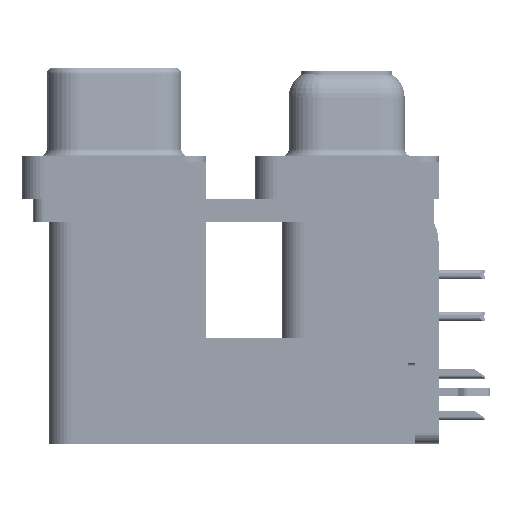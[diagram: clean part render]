
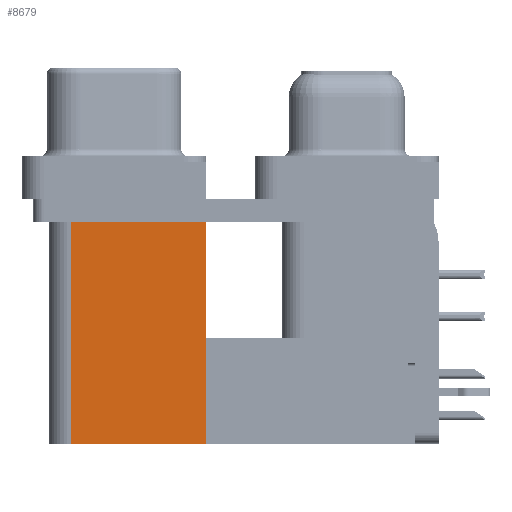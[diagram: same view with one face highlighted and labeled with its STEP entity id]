
A CAD part, left-side view. The second image highlights one B-rep face of the part: STEP entity #8679.
In plain terms, the highlighted planar face has unit normal (-1, 0, 0).
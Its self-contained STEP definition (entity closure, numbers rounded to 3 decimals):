
#277 = CARTESIAN_POINT ( 'NONE',  ( 3.79, 9.6, -2.5 ) ) ;
#1597 = AXIS2_PLACEMENT_3D ( 'NONE', #58110, #9900, #31339 ) ;
#2740 = ORIENTED_EDGE ( 'NONE', *, *, #32644, .F. ) ;
#8679 = ADVANCED_FACE ( 'NONE', ( #29939 ), #62696, .F. ) ;
#9900 = DIRECTION ( 'NONE',  ( 1., 0., 0. ) ) ;
#10101 = DIRECTION ( 'NONE',  ( 0., 1., 0. ) ) ;
#11709 = EDGE_CURVE ( 'NONE', #26536, #34856, #37534, .T. ) ;
#14113 = CARTESIAN_POINT ( 'NONE',  ( 3.79, 9.6, -2.5 ) ) ;
#20855 = VECTOR ( 'NONE', #66719, 1000. ) ;
#23496 = CARTESIAN_POINT ( 'NONE',  ( 3.79, 9.6, -19.2 ) ) ;
#23754 = LINE ( 'NONE', #45226, #20855 ) ;
#26536 = VERTEX_POINT ( 'NONE', #14113 ) ;
#27527 = EDGE_CURVE ( 'NONE', #42668, #34856, #57118, .T. ) ;
#29939 = FACE_OUTER_BOUND ( 'NONE', #42204, .T. ) ;
#31339 = DIRECTION ( 'NONE',  ( 0., 0., -1. ) ) ;
#31497 = EDGE_CURVE ( 'NONE', #40873, #26536, #32161, .T. ) ;
#32161 = LINE ( 'NONE', #53629, #51029 ) ;
#32644 = EDGE_CURVE ( 'NONE', #40873, #42668, #23754, .T. ) ;
#33054 = CARTESIAN_POINT ( 'NONE',  ( 3.79, 18.8, -2.5 ) ) ;
#34856 = VERTEX_POINT ( 'NONE', #33054 ) ;
#37534 = LINE ( 'NONE', #277, #57627 ) ;
#40873 = VERTEX_POINT ( 'NONE', #23496 ) ;
#42001 = ORIENTED_EDGE ( 'NONE', *, *, #11709, .T. ) ;
#42204 = EDGE_LOOP ( 'NONE', ( #42001, #47281, #2740, #51190 ) ) ;
#42366 = DIRECTION ( 'NONE',  ( 0., 0., 1. ) ) ;
#42668 = VERTEX_POINT ( 'NONE', #50528 ) ;
#45226 = CARTESIAN_POINT ( 'NONE',  ( 3.79, 9.6, -19.2 ) ) ;
#47281 = ORIENTED_EDGE ( 'NONE', *, *, #27527, .F. ) ;
#50528 = CARTESIAN_POINT ( 'NONE',  ( 3.79, 18.8, -19.2 ) ) ;
#51029 = VECTOR ( 'NONE', #42366, 1000. ) ;
#51190 = ORIENTED_EDGE ( 'NONE', *, *, #31497, .T. ) ;
#53629 = CARTESIAN_POINT ( 'NONE',  ( 3.79, 9.6, -19.2 ) ) ;
#56775 = CARTESIAN_POINT ( 'NONE',  ( 3.79, 18.8, -19.2 ) ) ;
#57118 = LINE ( 'NONE', #56775, #60935 ) ;
#57627 = VECTOR ( 'NONE', #10101, 1000. ) ;
#58110 = CARTESIAN_POINT ( 'NONE',  ( 3.79, 9.6, -19.2 ) ) ;
#60935 = VECTOR ( 'NONE', #68401, 1000. ) ;
#62696 = PLANE ( 'NONE',  #1597 ) ;
#66719 = DIRECTION ( 'NONE',  ( 0., 1., 0. ) ) ;
#68401 = DIRECTION ( 'NONE',  ( 0., 0., 1. ) ) ;
